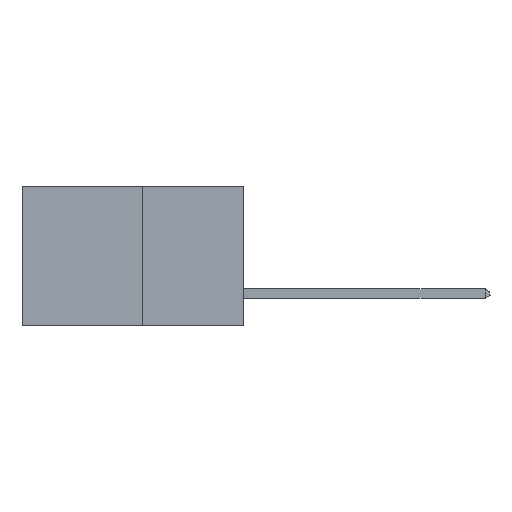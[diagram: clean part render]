
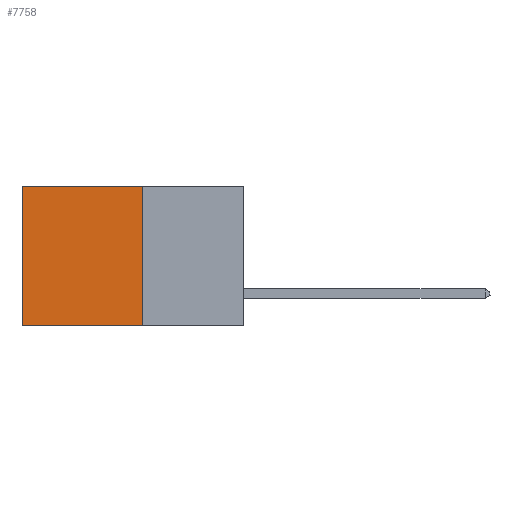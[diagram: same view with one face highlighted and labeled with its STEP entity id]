
A CAD part, left-side view. The second image highlights one B-rep face of the part: STEP entity #7758.
In plain terms, the highlighted planar face has unit normal (-1, 0, 0).
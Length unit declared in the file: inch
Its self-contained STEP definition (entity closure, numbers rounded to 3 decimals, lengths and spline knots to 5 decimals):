
#1 = DIRECTION ( 'NONE',  ( 0., 0., -1. ) ) ;
#26 = DIRECTION ( 'NONE',  ( 1., 0., 0. ) ) ;
#56 = PLANE ( 'NONE',  #7014 ) ;
#199 = EDGE_CURVE ( 'NONE', #317, #9318, #8032, .T. ) ;
#220 = CARTESIAN_POINT ( 'NONE',  ( 0.277, 0.27, -0.37 ) ) ;
#258 = VECTOR ( 'NONE', #5265, 39.37008 ) ;
#317 = VERTEX_POINT ( 'NONE', #5494 ) ;
#505 = DIRECTION ( 'NONE',  ( 0., 0., -1. ) ) ;
#928 = EDGE_CURVE ( 'NONE', #9752, #3484, #9490, .T. ) ;
#1937 = CARTESIAN_POINT ( 'NONE',  ( 0.277, 0.27, 0. ) ) ;
#2483 = ORIENTED_EDGE ( 'NONE', *, *, #928, .F. ) ;
#3347 = VECTOR ( 'NONE', #6339, 39.37008 ) ;
#3484 = VERTEX_POINT ( 'NONE', #7392 ) ;
#3512 = CARTESIAN_POINT ( 'NONE',  ( 0.277, 0.27, -0.37 ) ) ;
#3842 = VECTOR ( 'NONE', #505, 39.37008 ) ;
#3977 = ORIENTED_EDGE ( 'NONE', *, *, #5639, .T. ) ;
#3983 = VECTOR ( 'NONE', #5385, 39.37008 ) ;
#4235 = LINE ( 'NONE', #5171, #3983 ) ;
#5171 = CARTESIAN_POINT ( 'NONE',  ( 0.277, 0.27, 0. ) ) ;
#5265 = DIRECTION ( 'NONE',  ( 0., 1., 0. ) ) ;
#5385 = DIRECTION ( 'NONE',  ( 0., 1., 0. ) ) ;
#5494 = CARTESIAN_POINT ( 'NONE',  ( 0.277, 0.59, 0. ) ) ;
#5531 = CARTESIAN_POINT ( 'NONE',  ( 0.277, 0.27, -0.37 ) ) ;
#5639 = EDGE_CURVE ( 'NONE', #9752, #317, #4235, .T. ) ;
#5725 = ORIENTED_EDGE ( 'NONE', *, *, #199, .T. ) ;
#6243 = ORIENTED_EDGE ( 'NONE', *, *, #6252, .F. ) ;
#6252 = EDGE_CURVE ( 'NONE', #3484, #9318, #6767, .T. ) ;
#6339 = DIRECTION ( 'NONE',  ( 0., 0., -1. ) ) ;
#6767 = LINE ( 'NONE', #5531, #258 ) ;
#7014 = AXIS2_PLACEMENT_3D ( 'NONE', #220, #26, #1 ) ;
#7204 = CARTESIAN_POINT ( 'NONE',  ( 0.277, 0.59, -0.37 ) ) ;
#7392 = CARTESIAN_POINT ( 'NONE',  ( 0.277, 0.27, -0.37 ) ) ;
#7758 = ADVANCED_FACE ( 'NONE', ( #7836 ), #56, .F. ) ;
#7836 = FACE_OUTER_BOUND ( 'NONE', #9681, .T. ) ;
#8032 = LINE ( 'NONE', #8411, #3842 ) ;
#8411 = CARTESIAN_POINT ( 'NONE',  ( 0.277, 0.59, -0.37 ) ) ;
#9318 = VERTEX_POINT ( 'NONE', #7204 ) ;
#9490 = LINE ( 'NONE', #3512, #3347 ) ;
#9681 = EDGE_LOOP ( 'NONE', ( #5725, #6243, #2483, #3977 ) ) ;
#9752 = VERTEX_POINT ( 'NONE', #1937 ) ;
